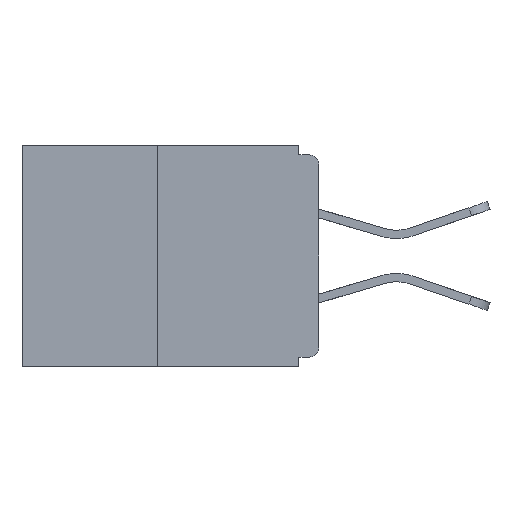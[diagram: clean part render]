
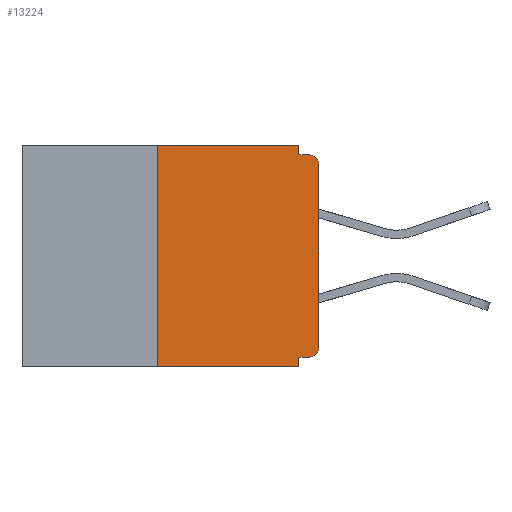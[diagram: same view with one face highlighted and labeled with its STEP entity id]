
A CAD part, left-side view. The second image highlights one B-rep face of the part: STEP entity #13224.
In plain terms, the highlighted planar face has unit normal (-1, 0, 0).
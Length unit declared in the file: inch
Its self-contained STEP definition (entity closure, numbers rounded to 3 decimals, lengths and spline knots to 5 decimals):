
#139 = EDGE_CURVE ( 'NONE', #4741, #16000, #580, .T. ) ;
#264 = LINE ( 'NONE', #16499, #3589 ) ;
#287 = CARTESIAN_POINT ( 'NONE',  ( 0., 0., -0.313 ) ) ;
#580 = LINE ( 'NONE', #17845, #8176 ) ;
#705 = EDGE_CURVE ( 'NONE', #11431, #19441, #8162, .T. ) ;
#794 = CARTESIAN_POINT ( 'NONE',  ( 0., 0.25, -0.343 ) ) ;
#1075 = EDGE_CURVE ( 'NONE', #7550, #2454, #16921, .T. ) ;
#1415 = CIRCLE ( 'NONE', #13438, 0.015 ) ;
#1476 = ORIENTED_EDGE ( 'NONE', *, *, #1075, .F. ) ;
#1615 = VECTOR ( 'NONE', #13956, 39.37008 ) ;
#1659 = DIRECTION ( 'NONE',  ( 0., 0., -1. ) ) ;
#1800 = CARTESIAN_POINT ( 'NONE',  ( 0., 0.25, 0. ) ) ;
#2052 = FACE_OUTER_BOUND ( 'NONE', #15033, .T. ) ;
#2235 = VERTEX_POINT ( 'NONE', #287 ) ;
#2454 = VERTEX_POINT ( 'NONE', #13612 ) ;
#2668 = DIRECTION ( 'NONE',  ( 0., -1., 0. ) ) ;
#2686 = CARTESIAN_POINT ( 'NONE',  ( 0., 0.015, -0.328 ) ) ;
#2736 = LINE ( 'NONE', #17982, #11301 ) ;
#2886 = CARTESIAN_POINT ( 'NONE',  ( 0., 0.015, -0.313 ) ) ;
#3537 = EDGE_CURVE ( 'NONE', #8462, #11431, #17519, .T. ) ;
#3589 = VECTOR ( 'NONE', #9112, 39.37008 ) ;
#4002 = VECTOR ( 'NONE', #2668, 39.37008 ) ;
#4093 = CARTESIAN_POINT ( 'NONE',  ( 0., 0.46, -0.343 ) ) ;
#4310 = ORIENTED_EDGE ( 'NONE', *, *, #12169, .T. ) ;
#4545 = CARTESIAN_POINT ( 'NONE',  ( 0., 0.031, -0.343 ) ) ;
#4741 = VERTEX_POINT ( 'NONE', #2686 ) ;
#5050 = VECTOR ( 'NONE', #15942, 39.37008 ) ;
#5300 = DIRECTION ( 'NONE',  ( 0., -1., 0. ) ) ;
#5791 = CARTESIAN_POINT ( 'NONE',  ( 0., 0., 0. ) ) ;
#5820 = DIRECTION ( 'NONE',  ( 0., 0., 1. ) ) ;
#6283 = ORIENTED_EDGE ( 'NONE', *, *, #10190, .F. ) ;
#6301 = ORIENTED_EDGE ( 'NONE', *, *, #10471, .T. ) ;
#6617 = CARTESIAN_POINT ( 'NONE',  ( 0., 0.46, 0. ) ) ;
#6758 = CARTESIAN_POINT ( 'NONE',  ( 0., 0.46, 0. ) ) ;
#7043 = DIRECTION ( 'NONE',  ( 0., 1., 0. ) ) ;
#7332 = DIRECTION ( 'NONE',  ( -1., 0., 0. ) ) ;
#7550 = VERTEX_POINT ( 'NONE', #14093 ) ;
#7855 = CARTESIAN_POINT ( 'NONE',  ( 0., 0., -0.03 ) ) ;
#8032 = LINE ( 'NONE', #4093, #4002 ) ;
#8162 = LINE ( 'NONE', #6617, #12199 ) ;
#8176 = VECTOR ( 'NONE', #7043, 39.37008 ) ;
#8368 = DIRECTION ( 'NONE',  ( 0., 0., -1. ) ) ;
#8462 = VERTEX_POINT ( 'NONE', #794 ) ;
#9112 = DIRECTION ( 'NONE',  ( 0., 0., -1. ) ) ;
#9181 = CIRCLE ( 'NONE', #16017, 0.015 ) ;
#9191 = EDGE_CURVE ( 'NONE', #8462, #11393, #8032, .T. ) ;
#9871 = CARTESIAN_POINT ( 'NONE',  ( 0., 0., -0.015 ) ) ;
#10190 = EDGE_CURVE ( 'NONE', #19441, #7550, #2736, .T. ) ;
#10223 = ORIENTED_EDGE ( 'NONE', *, *, #3537, .F. ) ;
#10471 = EDGE_CURVE ( 'NONE', #4741, #2235, #9181, .T. ) ;
#11301 = VECTOR ( 'NONE', #1659, 39.37008 ) ;
#11393 = VERTEX_POINT ( 'NONE', #4545 ) ;
#11404 = DIRECTION ( 'NONE',  ( 1., 0., 0. ) ) ;
#11431 = VERTEX_POINT ( 'NONE', #18128 ) ;
#12052 = CARTESIAN_POINT ( 'NONE',  ( 0., 0.015, -0.03 ) ) ;
#12169 = EDGE_CURVE ( 'NONE', #2235, #17913, #16811, .T. ) ;
#12199 = VECTOR ( 'NONE', #5300, 39.37008 ) ;
#12756 = AXIS2_PLACEMENT_3D ( 'NONE', #6758, #11404, #8368 ) ;
#12814 = PLANE ( 'NONE',  #12756 ) ;
#13224 = ADVANCED_FACE ( 'NONE', ( #2052 ), #12814, .F. ) ;
#13438 = AXIS2_PLACEMENT_3D ( 'NONE', #12052, #7332, #15029 ) ;
#13612 = CARTESIAN_POINT ( 'NONE',  ( 0., 0.015, -0.015 ) ) ;
#13750 = ORIENTED_EDGE ( 'NONE', *, *, #139, .F. ) ;
#13889 = ORIENTED_EDGE ( 'NONE', *, *, #17370, .T. ) ;
#13956 = DIRECTION ( 'NONE',  ( 0., 0., 1. ) ) ;
#14093 = CARTESIAN_POINT ( 'NONE',  ( 0., 0.031, -0.015 ) ) ;
#15029 = DIRECTION ( 'NONE',  ( 0., 0., -1. ) ) ;
#15033 = EDGE_LOOP ( 'NONE', ( #17711, #10223, #18745, #18726, #13750, #6301, #4310, #13889, #1476, #6283 ) ) ;
#15942 = DIRECTION ( 'NONE',  ( 0., -1., 0. ) ) ;
#16000 = VERTEX_POINT ( 'NONE', #16554 ) ;
#16017 = AXIS2_PLACEMENT_3D ( 'NONE', #2886, #17891, #17828 ) ;
#16499 = CARTESIAN_POINT ( 'NONE',  ( 0., 0.031, -0.343 ) ) ;
#16554 = CARTESIAN_POINT ( 'NONE',  ( 0., 0.031, -0.328 ) ) ;
#16572 = VECTOR ( 'NONE', #5820, 39.37008 ) ;
#16811 = LINE ( 'NONE', #5791, #16572 ) ;
#16921 = LINE ( 'NONE', #9871, #5050 ) ;
#17370 = EDGE_CURVE ( 'NONE', #17913, #2454, #1415, .T. ) ;
#17519 = LINE ( 'NONE', #1800, #1615 ) ;
#17711 = ORIENTED_EDGE ( 'NONE', *, *, #705, .F. ) ;
#17828 = DIRECTION ( 'NONE',  ( 0., 0., -1. ) ) ;
#17845 = CARTESIAN_POINT ( 'NONE',  ( 0., 0., -0.328 ) ) ;
#17891 = DIRECTION ( 'NONE',  ( -1., 0., 0. ) ) ;
#17913 = VERTEX_POINT ( 'NONE', #7855 ) ;
#17982 = CARTESIAN_POINT ( 'NONE',  ( 0., 0.031, 0. ) ) ;
#18128 = CARTESIAN_POINT ( 'NONE',  ( 0., 0.25, 0. ) ) ;
#18252 = EDGE_CURVE ( 'NONE', #16000, #11393, #264, .T. ) ;
#18273 = CARTESIAN_POINT ( 'NONE',  ( 0., 0.031, 0. ) ) ;
#18726 = ORIENTED_EDGE ( 'NONE', *, *, #18252, .F. ) ;
#18745 = ORIENTED_EDGE ( 'NONE', *, *, #9191, .T. ) ;
#19441 = VERTEX_POINT ( 'NONE', #18273 ) ;
